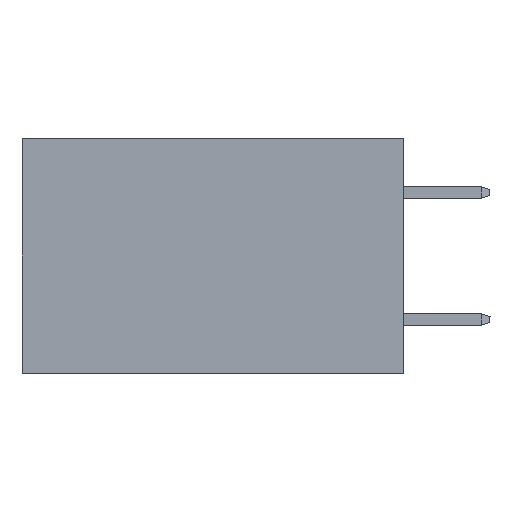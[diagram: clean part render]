
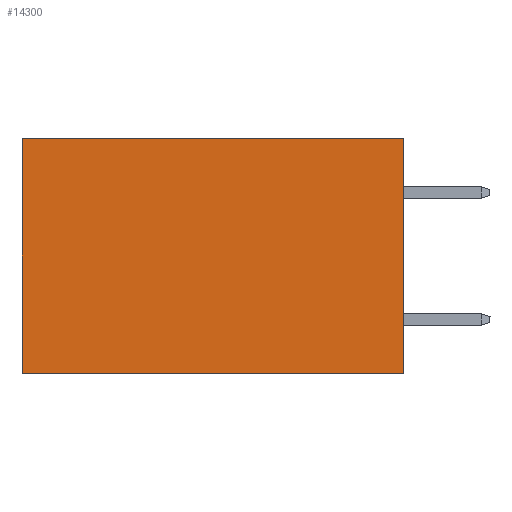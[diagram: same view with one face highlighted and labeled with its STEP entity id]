
A CAD part, left-side view. The second image highlights one B-rep face of the part: STEP entity #14300.
In plain terms, the highlighted planar face has unit normal (-1, 0, 0).
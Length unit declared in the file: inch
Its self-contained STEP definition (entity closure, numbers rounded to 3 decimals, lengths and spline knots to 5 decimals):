
#14 = VECTOR ( 'NONE', #21711, 39.37008 ) ;
#628 = LINE ( 'NONE', #27428, #29281 ) ;
#1221 = VERTEX_POINT ( 'NONE', #20044 ) ;
#2149 = FACE_OUTER_BOUND ( 'NONE', #2371, .T. ) ;
#2371 = EDGE_LOOP ( 'NONE', ( #3115, #3027, #9306, #24301 ) ) ;
#3027 = ORIENTED_EDGE ( 'NONE', *, *, #35386, .F. ) ;
#3115 = ORIENTED_EDGE ( 'NONE', *, *, #17785, .T. ) ;
#4163 = CARTESIAN_POINT ( 'NONE',  ( 0.2875, 0., -0.37 ) ) ;
#5340 = CARTESIAN_POINT ( 'NONE',  ( 0.2875, 0., 0. ) ) ;
#6538 = CARTESIAN_POINT ( 'NONE',  ( 0.2875, 0., 0. ) ) ;
#6716 = CARTESIAN_POINT ( 'NONE',  ( 0.2875, 0.6, 0. ) ) ;
#7398 = EDGE_CURVE ( 'NONE', #16151, #32870, #10275, .T. ) ;
#8362 = DIRECTION ( 'NONE',  ( 0., 0., -1. ) ) ;
#9306 = ORIENTED_EDGE ( 'NONE', *, *, #15790, .F. ) ;
#10134 = DIRECTION ( 'NONE',  ( 0., 0., -1. ) ) ;
#10275 = LINE ( 'NONE', #29755, #37169 ) ;
#14300 = ADVANCED_FACE ( 'NONE', ( #2149 ), #31223, .F. ) ;
#15790 = EDGE_CURVE ( 'NONE', #16151, #35915, #33223, .T. ) ;
#16151 = VERTEX_POINT ( 'NONE', #6538 ) ;
#16853 = DIRECTION ( 'NONE',  ( 1., 0., 0. ) ) ;
#16964 = LINE ( 'NONE', #4163, #14 ) ;
#17785 = EDGE_CURVE ( 'NONE', #32870, #1221, #628, .T. ) ;
#18932 = VECTOR ( 'NONE', #10134, 39.37008 ) ;
#19020 = CARTESIAN_POINT ( 'NONE',  ( 0.2875, 0., 0. ) ) ;
#20044 = CARTESIAN_POINT ( 'NONE',  ( 0.2875, 0.6, -0.37 ) ) ;
#20661 = AXIS2_PLACEMENT_3D ( 'NONE', #5340, #16853, #8362 ) ;
#21711 = DIRECTION ( 'NONE',  ( 0., 1., 0. ) ) ;
#24301 = ORIENTED_EDGE ( 'NONE', *, *, #7398, .T. ) ;
#27311 = DIRECTION ( 'NONE',  ( 0., 1., 0. ) ) ;
#27428 = CARTESIAN_POINT ( 'NONE',  ( 0.2875, 0.6, 0. ) ) ;
#29281 = VECTOR ( 'NONE', #35775, 39.37008 ) ;
#29755 = CARTESIAN_POINT ( 'NONE',  ( 0.2875, 0., 0. ) ) ;
#31223 = PLANE ( 'NONE',  #20661 ) ;
#32870 = VERTEX_POINT ( 'NONE', #6716 ) ;
#33223 = LINE ( 'NONE', #19020, #18932 ) ;
#34953 = CARTESIAN_POINT ( 'NONE',  ( 0.2875, 0., -0.37 ) ) ;
#35386 = EDGE_CURVE ( 'NONE', #35915, #1221, #16964, .T. ) ;
#35775 = DIRECTION ( 'NONE',  ( 0., 0., -1. ) ) ;
#35915 = VERTEX_POINT ( 'NONE', #34953 ) ;
#37169 = VECTOR ( 'NONE', #27311, 39.37008 ) ;
